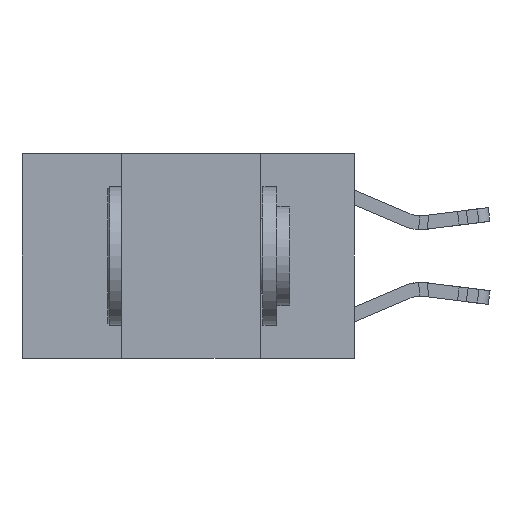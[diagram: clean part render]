
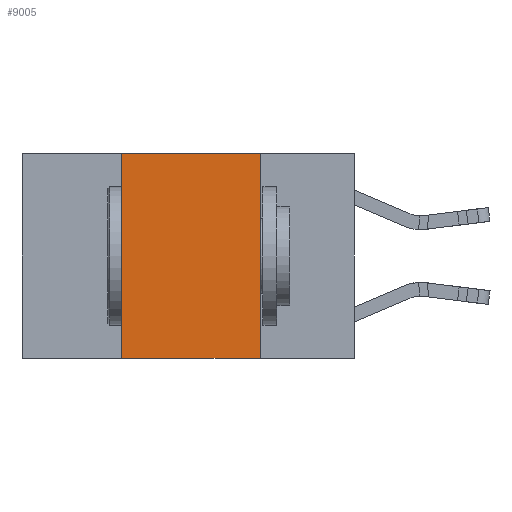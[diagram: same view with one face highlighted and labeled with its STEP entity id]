
A CAD part, left-side view. The second image highlights one B-rep face of the part: STEP entity #9005.
In plain terms, the highlighted planar face has unit normal (-1, 0, 0).
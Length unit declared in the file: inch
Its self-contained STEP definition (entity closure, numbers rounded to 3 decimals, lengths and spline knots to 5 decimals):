
#398 = DIRECTION ( 'NONE',  ( 0., -1., 0. ) ) ;
#637 = ORIENTED_EDGE ( 'NONE', *, *, #20979, .F. ) ;
#2330 = LINE ( 'NONE', #8870, #22994 ) ;
#2389 = CARTESIAN_POINT ( 'NONE',  ( 0., 0.6, -0.37 ) ) ;
#2406 = DIRECTION ( 'NONE',  ( 0., -1., 0. ) ) ;
#3683 = DIRECTION ( 'NONE',  ( 1., 0., 0. ) ) ;
#3778 = VERTEX_POINT ( 'NONE', #6380 ) ;
#4529 = CARTESIAN_POINT ( 'NONE',  ( 0., 0.17, -0.37 ) ) ;
#5273 = CARTESIAN_POINT ( 'NONE',  ( 0., 0.17, 0. ) ) ;
#5314 = VERTEX_POINT ( 'NONE', #26098 ) ;
#5777 = ORIENTED_EDGE ( 'NONE', *, *, #25375, .F. ) ;
#5966 = AXIS2_PLACEMENT_3D ( 'NONE', #19645, #3683, #26950 ) ;
#6380 = CARTESIAN_POINT ( 'NONE',  ( 0., 0.42, 0. ) ) ;
#7036 = CARTESIAN_POINT ( 'NONE',  ( 0., 0.42, -0.37 ) ) ;
#8084 = FACE_OUTER_BOUND ( 'NONE', #17860, .T. ) ;
#8759 = EDGE_CURVE ( 'NONE', #24390, #3778, #2330, .T. ) ;
#8870 = CARTESIAN_POINT ( 'NONE',  ( 0., 0.42, 0. ) ) ;
#9005 = ADVANCED_FACE ( 'NONE', ( #8084 ), #12807, .F. ) ;
#10030 = ORIENTED_EDGE ( 'NONE', *, *, #10190, .T. ) ;
#10190 = EDGE_CURVE ( 'NONE', #24390, #17627, #28374, .T. ) ;
#11648 = DIRECTION ( 'NONE',  ( 0., 0., -1. ) ) ;
#12807 = PLANE ( 'NONE',  #5966 ) ;
#13499 = VECTOR ( 'NONE', #11648, 39.37008 ) ;
#15877 = DIRECTION ( 'NONE',  ( 0., 0., 1. ) ) ;
#16694 = LINE ( 'NONE', #20937, #20406 ) ;
#17627 = VERTEX_POINT ( 'NONE', #4529 ) ;
#17860 = EDGE_LOOP ( 'NONE', ( #637, #5777, #29835, #10030 ) ) ;
#19645 = CARTESIAN_POINT ( 'NONE',  ( 0., 0.6, 0. ) ) ;
#20406 = VECTOR ( 'NONE', #2406, 39.37008 ) ;
#20937 = CARTESIAN_POINT ( 'NONE',  ( 0., 0.6, 0. ) ) ;
#20979 = EDGE_CURVE ( 'NONE', #5314, #17627, #23218, .T. ) ;
#22991 = VECTOR ( 'NONE', #398, 39.37008 ) ;
#22994 = VECTOR ( 'NONE', #15877, 39.37008 ) ;
#23218 = LINE ( 'NONE', #5273, #13499 ) ;
#24390 = VERTEX_POINT ( 'NONE', #7036 ) ;
#25375 = EDGE_CURVE ( 'NONE', #3778, #5314, #16694, .T. ) ;
#26098 = CARTESIAN_POINT ( 'NONE',  ( 0., 0.17, 0. ) ) ;
#26950 = DIRECTION ( 'NONE',  ( 0., 0., -1. ) ) ;
#28374 = LINE ( 'NONE', #2389, #22991 ) ;
#29835 = ORIENTED_EDGE ( 'NONE', *, *, #8759, .F. ) ;
